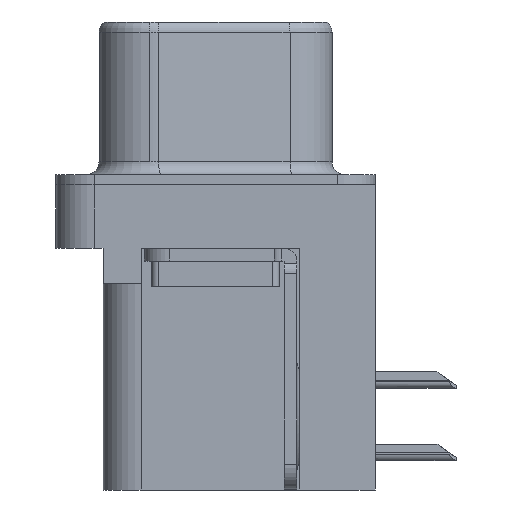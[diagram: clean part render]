
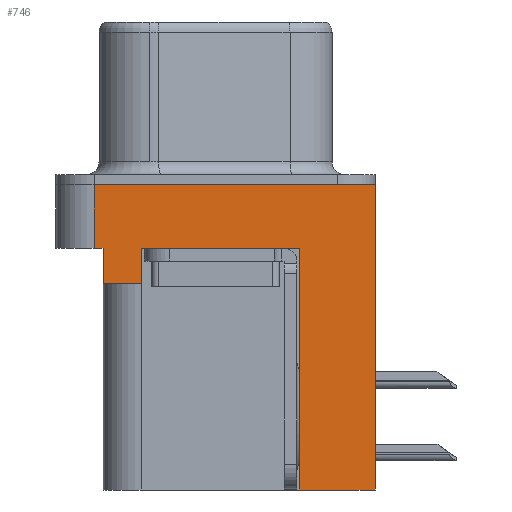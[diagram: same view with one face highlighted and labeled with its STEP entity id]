
A CAD part, left-side view. The second image highlights one B-rep face of the part: STEP entity #746.
In plain terms, the highlighted planar face has unit normal (-1, 0, 0).
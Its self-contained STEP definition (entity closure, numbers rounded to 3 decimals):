
#126 = CARTESIAN_POINT ( 'NONE',  ( -3., -6.275, 0. ) ) ;
#411 = ORIENTED_EDGE ( 'NONE', *, *, #23213, .F. ) ;
#527 = VECTOR ( 'NONE', #17600, 1000. ) ;
#602 = EDGE_CURVE ( 'NONE', #3875, #21899, #1073, .T. ) ;
#746 = ADVANCED_FACE ( 'NONE', ( #20925 ), #8849, .T. ) ;
#1073 = LINE ( 'NONE', #15689, #4096 ) ;
#1216 = EDGE_CURVE ( 'NONE', #8257, #13371, #19986, .T. ) ;
#1344 = VERTEX_POINT ( 'NONE', #17976 ) ;
#1379 = CARTESIAN_POINT ( 'NONE',  ( -3., -6.275, -2.5 ) ) ;
#1694 = DIRECTION ( 'NONE',  ( 0., 1., 0. ) ) ;
#1714 = CARTESIAN_POINT ( 'NONE',  ( -3., -3.295, -12. ) ) ;
#2565 = EDGE_CURVE ( 'NONE', #8257, #12419, #16941, .T. ) ;
#2824 = CARTESIAN_POINT ( 'NONE',  ( -3., -3.295, -12. ) ) ;
#2903 = ORIENTED_EDGE ( 'NONE', *, *, #15314, .F. ) ;
#2932 = DIRECTION ( 'NONE',  ( 0., 0., 1. ) ) ;
#3111 = LINE ( 'NONE', #1714, #14933 ) ;
#3154 = LINE ( 'NONE', #13284, #17661 ) ;
#3155 = ORIENTED_EDGE ( 'NONE', *, *, #1216, .T. ) ;
#3309 = VERTEX_POINT ( 'NONE', #126 ) ;
#3680 = EDGE_CURVE ( 'NONE', #6903, #11546, #12448, .T. ) ;
#3875 = VERTEX_POINT ( 'NONE', #22110 ) ;
#4096 = VECTOR ( 'NONE', #15856, 1000. ) ;
#4226 = DIRECTION ( 'NONE',  ( 0., 1., 0. ) ) ;
#4461 = CARTESIAN_POINT ( 'NONE',  ( -3., -3.295, -12. ) ) ;
#5218 = CARTESIAN_POINT ( 'NONE',  ( -3., 4.775, -2.5 ) ) ;
#6903 = VERTEX_POINT ( 'NONE', #12389 ) ;
#6947 = CARTESIAN_POINT ( 'NONE',  ( -3., -3.295, -2.5 ) ) ;
#7884 = CARTESIAN_POINT ( 'NONE',  ( -3., -6.275, -2.5 ) ) ;
#8257 = VERTEX_POINT ( 'NONE', #24494 ) ;
#8704 = DIRECTION ( 'NONE',  ( 0., 0., 1. ) ) ;
#8849 = PLANE ( 'NONE',  #13249 ) ;
#9354 = DIRECTION ( 'NONE',  ( 0., 0., 1. ) ) ;
#9871 = LINE ( 'NONE', #23177, #11319 ) ;
#9884 = VECTOR ( 'NONE', #8704, 1000. ) ;
#9952 = VECTOR ( 'NONE', #11333, 1000. ) ;
#10303 = EDGE_LOOP ( 'NONE', ( #14205, #23835, #3155, #411, #17453, #22041, #13421, #2903, #20040, #22372 ) ) ;
#10917 = EDGE_CURVE ( 'NONE', #21037, #3875, #9871, .T. ) ;
#11319 = VECTOR ( 'NONE', #19335, 1000. ) ;
#11333 = DIRECTION ( 'NONE',  ( 0., -1., 0. ) ) ;
#11441 = CARTESIAN_POINT ( 'NONE',  ( -3., 4.775, 0. ) ) ;
#11546 = VERTEX_POINT ( 'NONE', #2824 ) ;
#12389 = CARTESIAN_POINT ( 'NONE',  ( -3., -6.275, -12. ) ) ;
#12419 = VERTEX_POINT ( 'NONE', #11441 ) ;
#12421 = CARTESIAN_POINT ( 'NONE',  ( -3., 4.425, -3.9 ) ) ;
#12448 = LINE ( 'NONE', #4461, #19832 ) ;
#12465 = VECTOR ( 'NONE', #2932, 1000. ) ;
#13249 = AXIS2_PLACEMENT_3D ( 'NONE', #1379, #15088, #24254 ) ;
#13251 = LINE ( 'NONE', #7884, #527 ) ;
#13284 = CARTESIAN_POINT ( 'NONE',  ( -3., -6.275, 0. ) ) ;
#13371 = VERTEX_POINT ( 'NONE', #16335 ) ;
#13421 = ORIENTED_EDGE ( 'NONE', *, *, #602, .T. ) ;
#13513 = EDGE_CURVE ( 'NONE', #6903, #3309, #13251, .T. ) ;
#14002 = CARTESIAN_POINT ( 'NONE',  ( -3., 2.895, -3.9 ) ) ;
#14205 = ORIENTED_EDGE ( 'NONE', *, *, #14570, .F. ) ;
#14570 = EDGE_CURVE ( 'NONE', #12419, #3309, #3154, .T. ) ;
#14933 = VECTOR ( 'NONE', #9354, 1000. ) ;
#15088 = DIRECTION ( 'NONE',  ( -1., 0., 0. ) ) ;
#15314 = EDGE_CURVE ( 'NONE', #11546, #21899, #3111, .T. ) ;
#15689 = CARTESIAN_POINT ( 'NONE',  ( -3., -6.275, -2.5 ) ) ;
#15856 = DIRECTION ( 'NONE',  ( 0., -1., 0. ) ) ;
#16335 = CARTESIAN_POINT ( 'NONE',  ( -3., 4.425, -2.5 ) ) ;
#16941 = LINE ( 'NONE', #5218, #9884 ) ;
#17453 = ORIENTED_EDGE ( 'NONE', *, *, #24532, .F. ) ;
#17600 = DIRECTION ( 'NONE',  ( 0., 0., 1. ) ) ;
#17661 = VECTOR ( 'NONE', #22434, 1000. ) ;
#17976 = CARTESIAN_POINT ( 'NONE',  ( -3., 4.425, -3.9 ) ) ;
#18051 = CARTESIAN_POINT ( 'NONE',  ( -3., 4.425, -3.9 ) ) ;
#18107 = LINE ( 'NONE', #12421, #12465 ) ;
#19335 = DIRECTION ( 'NONE',  ( 0., 0., 1. ) ) ;
#19832 = VECTOR ( 'NONE', #4226, 1000. ) ;
#19986 = LINE ( 'NONE', #24288, #9952 ) ;
#20040 = ORIENTED_EDGE ( 'NONE', *, *, #3680, .F. ) ;
#20274 = VECTOR ( 'NONE', #1694, 1000. ) ;
#20925 = FACE_OUTER_BOUND ( 'NONE', #10303, .T. ) ;
#21037 = VERTEX_POINT ( 'NONE', #14002 ) ;
#21899 = VERTEX_POINT ( 'NONE', #6947 ) ;
#22041 = ORIENTED_EDGE ( 'NONE', *, *, #10917, .T. ) ;
#22053 = LINE ( 'NONE', #18051, #20274 ) ;
#22110 = CARTESIAN_POINT ( 'NONE',  ( -3., 2.895, -2.5 ) ) ;
#22372 = ORIENTED_EDGE ( 'NONE', *, *, #13513, .T. ) ;
#22434 = DIRECTION ( 'NONE',  ( 0., -1., 0. ) ) ;
#23177 = CARTESIAN_POINT ( 'NONE',  ( -3., 2.895, -3.9 ) ) ;
#23213 = EDGE_CURVE ( 'NONE', #1344, #13371, #18107, .T. ) ;
#23835 = ORIENTED_EDGE ( 'NONE', *, *, #2565, .F. ) ;
#24254 = DIRECTION ( 'NONE',  ( 0., 0., 1. ) ) ;
#24288 = CARTESIAN_POINT ( 'NONE',  ( -3., -6.275, -2.5 ) ) ;
#24494 = CARTESIAN_POINT ( 'NONE',  ( -3., 4.775, -2.5 ) ) ;
#24532 = EDGE_CURVE ( 'NONE', #21037, #1344, #22053, .T. ) ;
